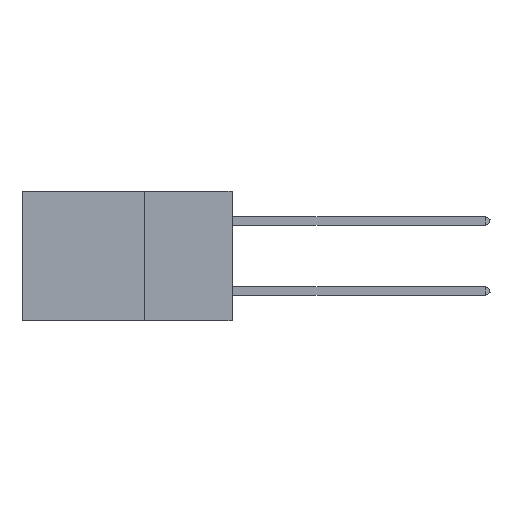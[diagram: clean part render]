
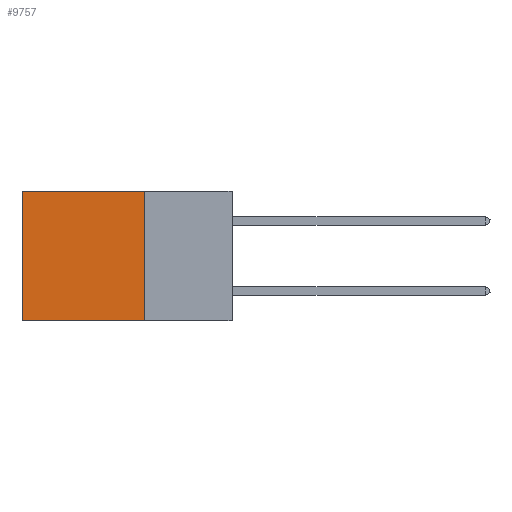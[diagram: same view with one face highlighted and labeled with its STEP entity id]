
A CAD part, left-side view. The second image highlights one B-rep face of the part: STEP entity #9757.
In plain terms, the highlighted planar face has unit normal (-1, 0, 0).
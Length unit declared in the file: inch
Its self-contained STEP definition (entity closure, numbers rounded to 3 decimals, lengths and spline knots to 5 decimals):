
#117 = EDGE_CURVE ( 'NONE', #24678, #445, #17033, .T. ) ;
#445 = VERTEX_POINT ( 'NONE', #7664 ) ;
#1052 = VECTOR ( 'NONE', #8951, 39.37008 ) ;
#1571 = DIRECTION ( 'NONE',  ( 1., 0., 0. ) ) ;
#1864 = CARTESIAN_POINT ( 'NONE',  ( 0.2875, 0.25, -0.37 ) ) ;
#2001 = ORIENTED_EDGE ( 'NONE', *, *, #2640, .F. ) ;
#2192 = CARTESIAN_POINT ( 'NONE',  ( 0.2875, 0.25, 0. ) ) ;
#2640 = EDGE_CURVE ( 'NONE', #36241, #445, #37207, .T. ) ;
#3054 = DIRECTION ( 'NONE',  ( 0., 1., 0. ) ) ;
#3568 = CARTESIAN_POINT ( 'NONE',  ( 0.2875, 0.25, 0. ) ) ;
#4461 = PLANE ( 'NONE',  #37997 ) ;
#6815 = VERTEX_POINT ( 'NONE', #24778 ) ;
#7472 = CARTESIAN_POINT ( 'NONE',  ( 0.2875, 0.25, 0. ) ) ;
#7664 = CARTESIAN_POINT ( 'NONE',  ( 0.2875, 0.6, -0.37 ) ) ;
#7780 = DIRECTION ( 'NONE',  ( 0., 1., 0. ) ) ;
#8611 = LINE ( 'NONE', #2192, #29210 ) ;
#8951 = DIRECTION ( 'NONE',  ( 0., 0., -1. ) ) ;
#9757 = ADVANCED_FACE ( 'NONE', ( #21330 ), #4461, .F. ) ;
#10340 = ORIENTED_EDGE ( 'NONE', *, *, #117, .T. ) ;
#10809 = ORIENTED_EDGE ( 'NONE', *, *, #34603, .T. ) ;
#15017 = VECTOR ( 'NONE', #3054, 39.37008 ) ;
#17033 = LINE ( 'NONE', #23635, #1052 ) ;
#17589 = VECTOR ( 'NONE', #7780, 39.37008 ) ;
#19784 = DIRECTION ( 'NONE',  ( 0., 0., -1. ) ) ;
#21101 = LINE ( 'NONE', #3568, #15017 ) ;
#21330 = FACE_OUTER_BOUND ( 'NONE', #28408, .T. ) ;
#22610 = CARTESIAN_POINT ( 'NONE',  ( 0.2875, 0.25, -0.37 ) ) ;
#23635 = CARTESIAN_POINT ( 'NONE',  ( 0.2875, 0.6, 0. ) ) ;
#24678 = VERTEX_POINT ( 'NONE', #26473 ) ;
#24778 = CARTESIAN_POINT ( 'NONE',  ( 0.2875, 0.25, 0. ) ) ;
#26473 = CARTESIAN_POINT ( 'NONE',  ( 0.2875, 0.6, 0. ) ) ;
#26676 = EDGE_CURVE ( 'NONE', #6815, #36241, #8611, .T. ) ;
#28408 = EDGE_LOOP ( 'NONE', ( #10340, #2001, #30473, #10809 ) ) ;
#28939 = DIRECTION ( 'NONE',  ( 0., 0., -1. ) ) ;
#29210 = VECTOR ( 'NONE', #19784, 39.37008 ) ;
#30473 = ORIENTED_EDGE ( 'NONE', *, *, #26676, .F. ) ;
#34603 = EDGE_CURVE ( 'NONE', #6815, #24678, #21101, .T. ) ;
#36241 = VERTEX_POINT ( 'NONE', #22610 ) ;
#37207 = LINE ( 'NONE', #1864, #17589 ) ;
#37997 = AXIS2_PLACEMENT_3D ( 'NONE', #7472, #1571, #28939 ) ;
